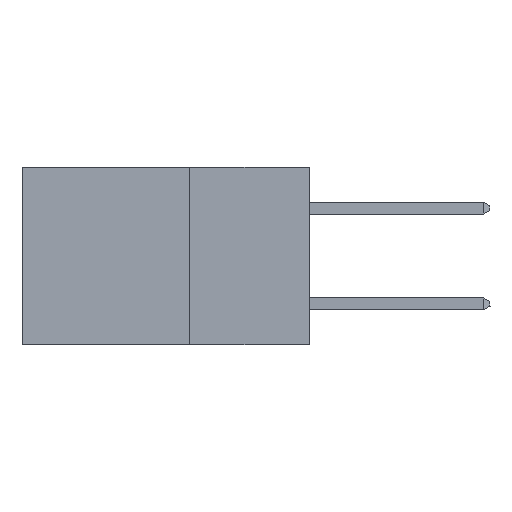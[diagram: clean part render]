
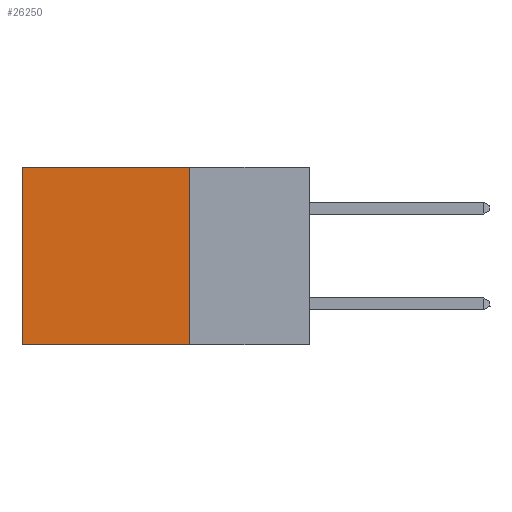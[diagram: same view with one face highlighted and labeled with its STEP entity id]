
A CAD part, left-side view. The second image highlights one B-rep face of the part: STEP entity #26250.
In plain terms, the highlighted planar face has unit normal (-1, 0, 0).
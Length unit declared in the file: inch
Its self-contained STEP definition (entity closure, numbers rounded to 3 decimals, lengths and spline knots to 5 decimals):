
#1336 = LINE ( 'NONE', #19765, #19949 ) ;
#1532 = AXIS2_PLACEMENT_3D ( 'NONE', #3766, #9657, #15574 ) ;
#3472 = ORIENTED_EDGE ( 'NONE', *, *, #34275, .F. ) ;
#3766 = CARTESIAN_POINT ( 'NONE',  ( 0.2875, 0.25, 0. ) ) ;
#7330 = EDGE_LOOP ( 'NONE', ( #35153, #3472, #22326, #27534 ) ) ;
#7590 = VECTOR ( 'NONE', #19980, 39.37008 ) ;
#7951 = EDGE_CURVE ( 'NONE', #12182, #27282, #34720, .T. ) ;
#8630 = FACE_OUTER_BOUND ( 'NONE', #7330, .T. ) ;
#9657 = DIRECTION ( 'NONE',  ( 1., 0., 0. ) ) ;
#10217 = VECTOR ( 'NONE', #23495, 39.37008 ) ;
#12182 = VERTEX_POINT ( 'NONE', #13824 ) ;
#12691 = CARTESIAN_POINT ( 'NONE',  ( 0.2875, 0.25, 0. ) ) ;
#13824 = CARTESIAN_POINT ( 'NONE',  ( 0.2875, 0.25, 0. ) ) ;
#13829 = CARTESIAN_POINT ( 'NONE',  ( 0.2875, 0.6, -0.37 ) ) ;
#13935 = DIRECTION ( 'NONE',  ( 0., 0., -1. ) ) ;
#15574 = DIRECTION ( 'NONE',  ( 0., 0., -1. ) ) ;
#15958 = VERTEX_POINT ( 'NONE', #13829 ) ;
#15959 = VECTOR ( 'NONE', #37312, 39.37008 ) ;
#17096 = EDGE_CURVE ( 'NONE', #12182, #30864, #31384, .T. ) ;
#17344 = PLANE ( 'NONE',  #1532 ) ;
#19765 = CARTESIAN_POINT ( 'NONE',  ( 0.2875, 0.6, 0. ) ) ;
#19949 = VECTOR ( 'NONE', #13935, 39.37008 ) ;
#19980 = DIRECTION ( 'NONE',  ( 0., 0., -1. ) ) ;
#22326 = ORIENTED_EDGE ( 'NONE', *, *, #7951, .F. ) ;
#23495 = DIRECTION ( 'NONE',  ( 0., 1., 0. ) ) ;
#26250 = ADVANCED_FACE ( 'NONE', ( #8630 ), #17344, .F. ) ;
#27282 = VERTEX_POINT ( 'NONE', #30981 ) ;
#27534 = ORIENTED_EDGE ( 'NONE', *, *, #17096, .T. ) ;
#29882 = CARTESIAN_POINT ( 'NONE',  ( 0.2875, 0.25, 0. ) ) ;
#30864 = VERTEX_POINT ( 'NONE', #32488 ) ;
#30981 = CARTESIAN_POINT ( 'NONE',  ( 0.2875, 0.25, -0.37 ) ) ;
#31384 = LINE ( 'NONE', #12691, #15959 ) ;
#32488 = CARTESIAN_POINT ( 'NONE',  ( 0.2875, 0.6, 0. ) ) ;
#34275 = EDGE_CURVE ( 'NONE', #27282, #15958, #35057, .T. ) ;
#34720 = LINE ( 'NONE', #29882, #7590 ) ;
#35057 = LINE ( 'NONE', #35363, #10217 ) ;
#35153 = ORIENTED_EDGE ( 'NONE', *, *, #37282, .T. ) ;
#35363 = CARTESIAN_POINT ( 'NONE',  ( 0.2875, 0.25, -0.37 ) ) ;
#37282 = EDGE_CURVE ( 'NONE', #30864, #15958, #1336, .T. ) ;
#37312 = DIRECTION ( 'NONE',  ( 0., 1., 0. ) ) ;
